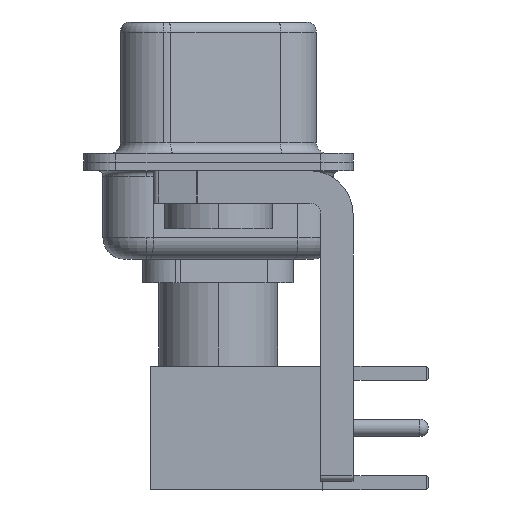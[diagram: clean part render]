
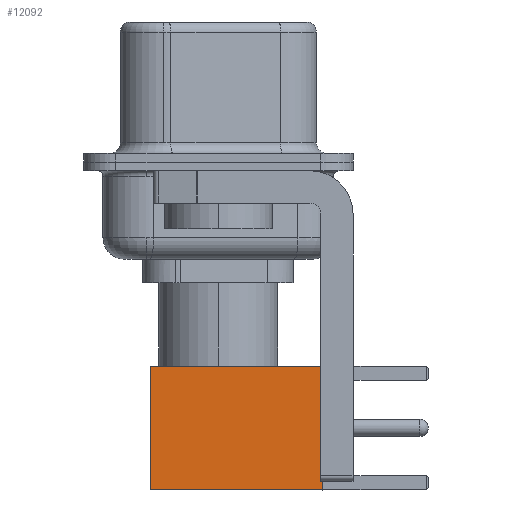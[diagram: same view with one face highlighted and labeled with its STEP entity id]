
A CAD part, left-side view. The second image highlights one B-rep face of the part: STEP entity #12092.
In plain terms, the highlighted face is planar.
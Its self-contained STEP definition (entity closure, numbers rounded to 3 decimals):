
#419 = DIRECTION ( 'NONE',  ( 0., 1., 0. ) ) ;
#1486 = AXIS2_PLACEMENT_3D ( 'NONE', #16514, #419, #20271 ) ;
#1789 = DIRECTION ( 'NONE',  ( 0., 0., -1. ) ) ;
#1952 = PLANE ( 'NONE',  #1486 ) ;
#2193 = DIRECTION ( 'NONE',  ( 0., 0., -1. ) ) ;
#2363 = VERTEX_POINT ( 'NONE', #10020 ) ;
#2964 = CARTESIAN_POINT ( 'NONE',  ( -2.875, 2.875, 0. ) ) ;
#3348 = LINE ( 'NONE', #8759, #13118 ) ;
#3435 = LINE ( 'NONE', #15775, #7514 ) ;
#4886 = VERTEX_POINT ( 'NONE', #2964 ) ;
#5638 = ORIENTED_EDGE ( 'NONE', *, *, #14363, .T. ) ;
#5943 = EDGE_CURVE ( 'NONE', #13748, #4886, #3348, .T. ) ;
#6883 = ORIENTED_EDGE ( 'NONE', *, *, #5943, .T. ) ;
#7514 = VECTOR ( 'NONE', #1789, 1000. ) ;
#8759 = CARTESIAN_POINT ( 'NONE',  ( 0., 2.875, 0. ) ) ;
#8876 = DIRECTION ( 'NONE',  ( -1., 0., 0. ) ) ;
#10020 = CARTESIAN_POINT ( 'NONE',  ( -2.875, 2.875, 8. ) ) ;
#10267 = CARTESIAN_POINT ( 'NONE',  ( 2.875, 2.875, 8. ) ) ;
#10862 = VECTOR ( 'NONE', #16141, 1000. ) ;
#11107 = FACE_OUTER_BOUND ( 'NONE', #11917, .T. ) ;
#11917 = EDGE_LOOP ( 'NONE', ( #5638, #6883, #20448, #21191 ) ) ;
#12092 = ADVANCED_FACE ( 'NONE', ( #11107 ), #1952, .T. ) ;
#12478 = EDGE_CURVE ( 'NONE', #2363, #4886, #19932, .T. ) ;
#13118 = VECTOR ( 'NONE', #8876, 1000. ) ;
#13748 = VERTEX_POINT ( 'NONE', #15447 ) ;
#13864 = EDGE_CURVE ( 'NONE', #21820, #2363, #17678, .T. ) ;
#14363 = EDGE_CURVE ( 'NONE', #21820, #13748, #3435, .T. ) ;
#14883 = CARTESIAN_POINT ( 'NONE',  ( -2.875, 2.875, 0. ) ) ;
#15447 = CARTESIAN_POINT ( 'NONE',  ( 2.875, 2.875, 0. ) ) ;
#15775 = CARTESIAN_POINT ( 'NONE',  ( 2.875, 2.875, 0. ) ) ;
#16032 = CARTESIAN_POINT ( 'NONE',  ( 0., 2.875, 8. ) ) ;
#16141 = DIRECTION ( 'NONE',  ( -1., 0., 0. ) ) ;
#16514 = CARTESIAN_POINT ( 'NONE',  ( 2.875, 2.875, 0. ) ) ;
#17678 = LINE ( 'NONE', #16032, #10862 ) ;
#19086 = VECTOR ( 'NONE', #2193, 1000. ) ;
#19932 = LINE ( 'NONE', #14883, #19086 ) ;
#20271 = DIRECTION ( 'NONE',  ( 0., 0., 1. ) ) ;
#20448 = ORIENTED_EDGE ( 'NONE', *, *, #12478, .F. ) ;
#21191 = ORIENTED_EDGE ( 'NONE', *, *, #13864, .F. ) ;
#21820 = VERTEX_POINT ( 'NONE', #10267 ) ;
